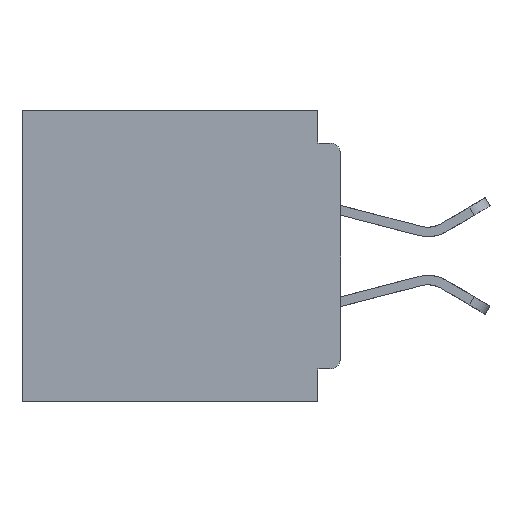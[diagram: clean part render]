
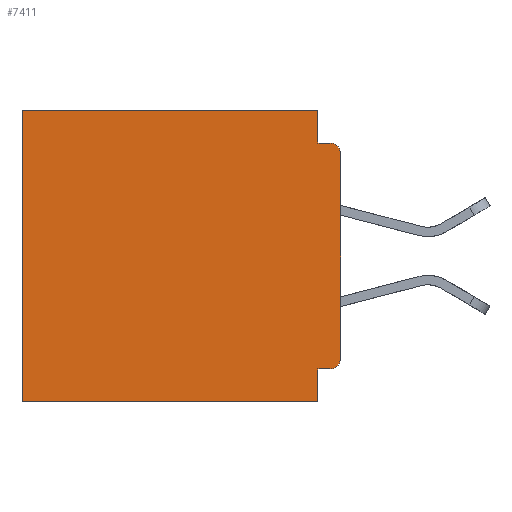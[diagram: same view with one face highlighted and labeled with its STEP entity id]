
A CAD part, left-side view. The second image highlights one B-rep face of the part: STEP entity #7411.
In plain terms, the highlighted planar face has unit normal (-1, 0, 0).
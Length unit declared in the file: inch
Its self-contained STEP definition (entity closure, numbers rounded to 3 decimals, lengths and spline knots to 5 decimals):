
#129 = DIRECTION ( 'NONE',  ( 0., 1., 0. ) ) ;
#367 = VECTOR ( 'NONE', #23581, 39.37008 ) ;
#394 = VERTEX_POINT ( 'NONE', #21394 ) ;
#586 = LINE ( 'NONE', #30888, #31137 ) ;
#627 = LINE ( 'NONE', #32260, #15514 ) ;
#787 = EDGE_CURVE ( 'NONE', #11282, #30250, #32711, .T. ) ;
#1156 = EDGE_CURVE ( 'NONE', #11282, #32072, #18021, .T. ) ;
#1800 = VERTEX_POINT ( 'NONE', #11611 ) ;
#2088 = VERTEX_POINT ( 'NONE', #36654 ) ;
#2161 = CARTESIAN_POINT ( 'NONE',  ( 0.3, 0.031, -0.355 ) ) ;
#2303 = ORIENTED_EDGE ( 'NONE', *, *, #37951, .T. ) ;
#2812 = DIRECTION ( 'NONE',  ( 0., 0., -1. ) ) ;
#2853 = VECTOR ( 'NONE', #129, 39.37008 ) ;
#3392 = EDGE_CURVE ( 'NONE', #15938, #33818, #627, .T. ) ;
#3819 = VECTOR ( 'NONE', #15968, 39.37008 ) ;
#4180 = ORIENTED_EDGE ( 'NONE', *, *, #16331, .F. ) ;
#4710 = CARTESIAN_POINT ( 'NONE',  ( 0.3, 0.031, 0. ) ) ;
#5873 = VECTOR ( 'NONE', #9804, 39.37008 ) ;
#6398 = LINE ( 'NONE', #12394, #15195 ) ;
#6969 = ORIENTED_EDGE ( 'NONE', *, *, #1156, .F. ) ;
#7411 = ADVANCED_FACE ( 'NONE', ( #25993 ), #34787, .F. ) ;
#7669 = CARTESIAN_POINT ( 'NONE',  ( 0.3, 0.031, 0. ) ) ;
#8342 = ORIENTED_EDGE ( 'NONE', *, *, #35506, .F. ) ;
#8636 = EDGE_CURVE ( 'NONE', #1800, #30205, #13728, .T. ) ;
#9804 = DIRECTION ( 'NONE',  ( 0., 0., -1. ) ) ;
#9809 = LINE ( 'NONE', #17973, #2853 ) ;
#9851 = EDGE_CURVE ( 'NONE', #32072, #25150, #586, .T. ) ;
#10226 = CARTESIAN_POINT ( 'NONE',  ( 0.3, 0.015, -0.045 ) ) ;
#11128 = CARTESIAN_POINT ( 'NONE',  ( 0.3, 0.031, -0.045 ) ) ;
#11282 = VERTEX_POINT ( 'NONE', #7669 ) ;
#11611 = CARTESIAN_POINT ( 'NONE',  ( 0.3, 0., -0.06 ) ) ;
#11727 = CARTESIAN_POINT ( 'NONE',  ( 0.3, 0.015, -0.34 ) ) ;
#12394 = CARTESIAN_POINT ( 'NONE',  ( 0.3, 0.437, -0.4 ) ) ;
#12678 = CARTESIAN_POINT ( 'NONE',  ( 0.3, 0., -0.4 ) ) ;
#13016 = CARTESIAN_POINT ( 'NONE',  ( 0.3, 0.031, -0.4 ) ) ;
#13728 = LINE ( 'NONE', #12678, #5873 ) ;
#14638 = DIRECTION ( 'NONE',  ( 0., 0., -1. ) ) ;
#15195 = VECTOR ( 'NONE', #32899, 39.37008 ) ;
#15496 = CARTESIAN_POINT ( 'NONE',  ( 0.3, 0., 0. ) ) ;
#15514 = VECTOR ( 'NONE', #26014, 39.37008 ) ;
#15938 = VERTEX_POINT ( 'NONE', #30860 ) ;
#15968 = DIRECTION ( 'NONE',  ( 0., 0., -1. ) ) ;
#16238 = ORIENTED_EDGE ( 'NONE', *, *, #8636, .F. ) ;
#16331 = EDGE_CURVE ( 'NONE', #394, #2088, #9809, .T. ) ;
#17082 = VECTOR ( 'NONE', #20174, 39.37008 ) ;
#17973 = CARTESIAN_POINT ( 'NONE',  ( 0.3, 0., -0.4 ) ) ;
#18021 = LINE ( 'NONE', #4710, #17082 ) ;
#20174 = DIRECTION ( 'NONE',  ( 0., 0., -1. ) ) ;
#20230 = EDGE_LOOP ( 'NONE', ( #16238, #26533, #24716, #6969, #21955, #2303, #4180, #8342, #35375, #33559 ) ) ;
#20697 = DIRECTION ( 'NONE',  ( -1., 0., 0. ) ) ;
#21394 = CARTESIAN_POINT ( 'NONE',  ( 0.3, 0.031, -0.4 ) ) ;
#21955 = ORIENTED_EDGE ( 'NONE', *, *, #787, .T. ) ;
#23025 = EDGE_CURVE ( 'NONE', #15938, #30205, #28875, .T. ) ;
#23581 = DIRECTION ( 'NONE',  ( 0., 1., 0. ) ) ;
#23971 = AXIS2_PLACEMENT_3D ( 'NONE', #11727, #32257, #14638 ) ;
#24716 = ORIENTED_EDGE ( 'NONE', *, *, #9851, .F. ) ;
#25150 = VERTEX_POINT ( 'NONE', #10226 ) ;
#25993 = FACE_OUTER_BOUND ( 'NONE', #20230, .T. ) ;
#26014 = DIRECTION ( 'NONE',  ( 0., 1., 0. ) ) ;
#26533 = ORIENTED_EDGE ( 'NONE', *, *, #29291, .T. ) ;
#28431 = CARTESIAN_POINT ( 'NONE',  ( 0.3, 0.437, 0. ) ) ;
#28875 = CIRCLE ( 'NONE', #23971, 0.015 ) ;
#29291 = EDGE_CURVE ( 'NONE', #1800, #25150, #36257, .T. ) ;
#29296 = LINE ( 'NONE', #13016, #3819 ) ;
#30205 = VERTEX_POINT ( 'NONE', #30909 ) ;
#30250 = VERTEX_POINT ( 'NONE', #28431 ) ;
#30860 = CARTESIAN_POINT ( 'NONE',  ( 0.3, 0.015, -0.355 ) ) ;
#30888 = CARTESIAN_POINT ( 'NONE',  ( 0.3, 0., -0.045 ) ) ;
#30909 = CARTESIAN_POINT ( 'NONE',  ( 0.3, 0., -0.34 ) ) ;
#31137 = VECTOR ( 'NONE', #33730, 39.37008 ) ;
#32017 = AXIS2_PLACEMENT_3D ( 'NONE', #37954, #20697, #2812 ) ;
#32072 = VERTEX_POINT ( 'NONE', #11128 ) ;
#32257 = DIRECTION ( 'NONE',  ( -1., 0., 0. ) ) ;
#32260 = CARTESIAN_POINT ( 'NONE',  ( 0.3, 0., -0.355 ) ) ;
#32711 = LINE ( 'NONE', #15496, #367 ) ;
#32899 = DIRECTION ( 'NONE',  ( 0., 0., -1. ) ) ;
#33559 = ORIENTED_EDGE ( 'NONE', *, *, #23025, .T. ) ;
#33730 = DIRECTION ( 'NONE',  ( 0., -1., 0. ) ) ;
#33818 = VERTEX_POINT ( 'NONE', #2161 ) ;
#34276 = DIRECTION ( 'NONE',  ( 0., 0., -1. ) ) ;
#34535 = DIRECTION ( 'NONE',  ( 1., 0., 0. ) ) ;
#34738 = CARTESIAN_POINT ( 'NONE',  ( 0.3, 0., -0.4 ) ) ;
#34786 = AXIS2_PLACEMENT_3D ( 'NONE', #34738, #34535, #34276 ) ;
#34787 = PLANE ( 'NONE',  #34786 ) ;
#35375 = ORIENTED_EDGE ( 'NONE', *, *, #3392, .F. ) ;
#35506 = EDGE_CURVE ( 'NONE', #33818, #394, #29296, .T. ) ;
#36257 = CIRCLE ( 'NONE', #32017, 0.015 ) ;
#36654 = CARTESIAN_POINT ( 'NONE',  ( 0.3, 0.437, -0.4 ) ) ;
#37951 = EDGE_CURVE ( 'NONE', #30250, #2088, #6398, .T. ) ;
#37954 = CARTESIAN_POINT ( 'NONE',  ( 0.3, 0.015, -0.06 ) ) ;
